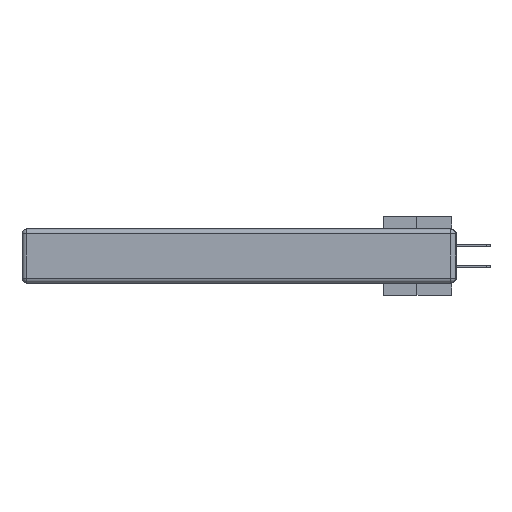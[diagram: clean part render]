
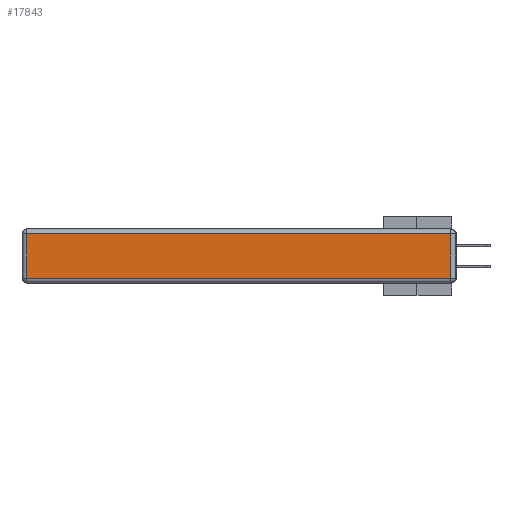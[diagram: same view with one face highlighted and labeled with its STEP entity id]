
A CAD part, left-side view. The second image highlights one B-rep face of the part: STEP entity #17843.
In plain terms, the highlighted planar face has unit normal (-1, 0, 0).
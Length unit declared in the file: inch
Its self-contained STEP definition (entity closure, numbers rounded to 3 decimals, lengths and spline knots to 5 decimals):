
#380 = CARTESIAN_POINT ( 'NONE',  ( 0., 0.03, -0.343 ) ) ;
#2306 = CARTESIAN_POINT ( 'NONE',  ( 0., 0.03, -0.03 ) ) ;
#2493 = DIRECTION ( 'NONE',  ( 0., 0., -1. ) ) ;
#3097 = DIRECTION ( 'NONE',  ( 0., 0., 1. ) ) ;
#4597 = LINE ( 'NONE', #9780, #20977 ) ;
#5639 = CARTESIAN_POINT ( 'NONE',  ( 0., 0.03, -0.313 ) ) ;
#6398 = LINE ( 'NONE', #24233, #20205 ) ;
#7572 = EDGE_LOOP ( 'NONE', ( #20914, #33807, #28903, #27221 ) ) ;
#9183 = LINE ( 'NONE', #380, #34137 ) ;
#9687 = CARTESIAN_POINT ( 'NONE',  ( 0., 2.72, -0.313 ) ) ;
#9780 = CARTESIAN_POINT ( 'NONE',  ( 0., 2.75, -0.03 ) ) ;
#11016 = AXIS2_PLACEMENT_3D ( 'NONE', #24623, #24868, #27753 ) ;
#11060 = CARTESIAN_POINT ( 'NONE',  ( 0., 2.72, -0.03 ) ) ;
#12067 = VERTEX_POINT ( 'NONE', #9687 ) ;
#13327 = VERTEX_POINT ( 'NONE', #11060 ) ;
#17843 = ADVANCED_FACE ( 'NONE', ( #25260 ), #30247, .T. ) ;
#18433 = DIRECTION ( 'NONE',  ( 0., 1., 0. ) ) ;
#18619 = VECTOR ( 'NONE', #2493, 39.37008 ) ;
#20205 = VECTOR ( 'NONE', #24722, 39.37008 ) ;
#20914 = ORIENTED_EDGE ( 'NONE', *, *, #31244, .T. ) ;
#20977 = VECTOR ( 'NONE', #18433, 39.37008 ) ;
#21896 = CARTESIAN_POINT ( 'NONE',  ( 0., 2.72, -0.343 ) ) ;
#22491 = LINE ( 'NONE', #21896, #18619 ) ;
#24233 = CARTESIAN_POINT ( 'NONE',  ( 0., 0., -0.313 ) ) ;
#24440 = VERTEX_POINT ( 'NONE', #2306 ) ;
#24623 = CARTESIAN_POINT ( 'NONE',  ( 0., 0., -0.343 ) ) ;
#24722 = DIRECTION ( 'NONE',  ( 0., -1., 0. ) ) ;
#24868 = DIRECTION ( 'NONE',  ( -1., 0., 0. ) ) ;
#25260 = FACE_OUTER_BOUND ( 'NONE', #7572, .T. ) ;
#27221 = ORIENTED_EDGE ( 'NONE', *, *, #35273, .T. ) ;
#27753 = DIRECTION ( 'NONE',  ( 0., 0., 1. ) ) ;
#28790 = EDGE_CURVE ( 'NONE', #30757, #24440, #9183, .T. ) ;
#28903 = ORIENTED_EDGE ( 'NONE', *, *, #32218, .T. ) ;
#30247 = PLANE ( 'NONE',  #11016 ) ;
#30757 = VERTEX_POINT ( 'NONE', #5639 ) ;
#31244 = EDGE_CURVE ( 'NONE', #12067, #30757, #6398, .T. ) ;
#32218 = EDGE_CURVE ( 'NONE', #24440, #13327, #4597, .T. ) ;
#33807 = ORIENTED_EDGE ( 'NONE', *, *, #28790, .T. ) ;
#34137 = VECTOR ( 'NONE', #3097, 39.37008 ) ;
#35273 = EDGE_CURVE ( 'NONE', #13327, #12067, #22491, .T. ) ;
